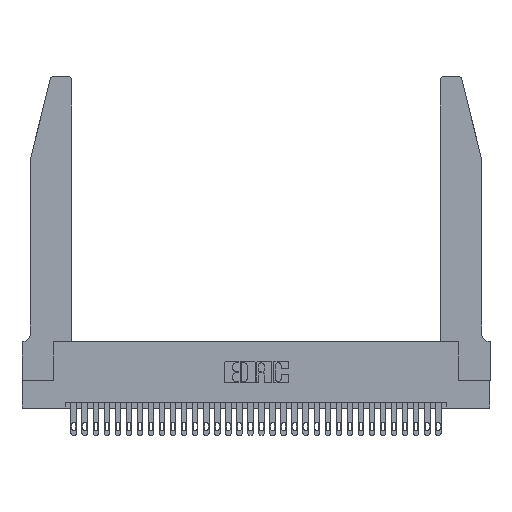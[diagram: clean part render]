
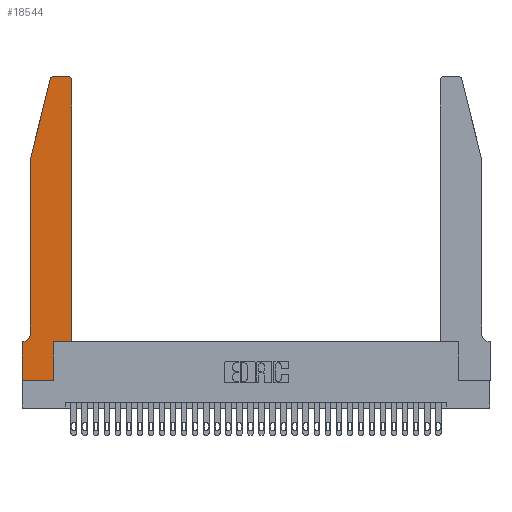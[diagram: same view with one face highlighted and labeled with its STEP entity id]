
A CAD part, top view. The second image highlights one B-rep face of the part: STEP entity #18544.
In plain terms, the highlighted planar face has unit normal (0, 0, 1).
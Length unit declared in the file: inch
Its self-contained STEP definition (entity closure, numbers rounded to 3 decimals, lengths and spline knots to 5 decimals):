
#25 = ORIENTED_EDGE ( 'NONE', *, *, #25476, .T. ) ;
#168 = AXIS2_PLACEMENT_3D ( 'NONE', #1321, #31661, #31769 ) ;
#271 = DIRECTION ( 'NONE',  ( 0., 0., 1. ) ) ;
#1321 = CARTESIAN_POINT ( 'NONE',  ( 0., 0.35, 0.37 ) ) ;
#1745 = VERTEX_POINT ( 'NONE', #8713 ) ;
#1858 = CARTESIAN_POINT ( 'NONE',  ( 0.4505, 2.72, 0.37 ) ) ;
#2359 = EDGE_CURVE ( 'NONE', #8991, #23060, #26266, .T. ) ;
#2499 = LINE ( 'NONE', #14988, #24441 ) ;
#2896 = ORIENTED_EDGE ( 'NONE', *, *, #8494, .T. ) ;
#3615 = DIRECTION ( 'NONE',  ( 1., 0., 0. ) ) ;
#3685 = ORIENTED_EDGE ( 'NONE', *, *, #18693, .T. ) ;
#4271 = CARTESIAN_POINT ( 'NONE',  ( 0.2605, 2.75, 0.37 ) ) ;
#4731 = VECTOR ( 'NONE', #11749, 39.37008 ) ;
#4778 = VERTEX_POINT ( 'NONE', #31301 ) ;
#5156 = CARTESIAN_POINT ( 'NONE',  ( 0.0055, 0.42, 0.37 ) ) ;
#6467 = CARTESIAN_POINT ( 'NONE',  ( 0.0755, 0.35, 0.37 ) ) ;
#7133 = CIRCLE ( 'NONE', #19119, 0.03 ) ;
#7186 = DIRECTION ( 'NONE',  ( 0., -1., 0. ) ) ;
#7257 = CARTESIAN_POINT ( 'NONE',  ( 0.2865, 0.35, 0.37 ) ) ;
#7269 = ORIENTED_EDGE ( 'NONE', *, *, #18301, .T. ) ;
#7534 = CARTESIAN_POINT ( 'NONE',  ( 0.4205, 2.72, 0.37 ) ) ;
#7924 = VERTEX_POINT ( 'NONE', #23741 ) ;
#8092 = CARTESIAN_POINT ( 'NONE',  ( 0.284, 2.72, 0.37 ) ) ;
#8243 = VERTEX_POINT ( 'NONE', #7257 ) ;
#8494 = EDGE_CURVE ( 'NONE', #1745, #23053, #29633, .T. ) ;
#8578 = AXIS2_PLACEMENT_3D ( 'NONE', #7534, #271, #14889 ) ;
#8713 = CARTESIAN_POINT ( 'NONE',  ( 0.0055, 0.35, 0.37 ) ) ;
#8819 = CARTESIAN_POINT ( 'NONE',  ( 0.4505, 0.35, 0.37 ) ) ;
#8991 = VERTEX_POINT ( 'NONE', #28957 ) ;
#9168 = ORIENTED_EDGE ( 'NONE', *, *, #27888, .T. ) ;
#9674 = CIRCLE ( 'NONE', #29770, 0.07 ) ;
#10030 = FACE_OUTER_BOUND ( 'NONE', #10516, .T. ) ;
#10516 = EDGE_LOOP ( 'NONE', ( #11711, #15604, #7269, #23834, #25, #2896, #9168, #18873, #19729, #15677, #13656, #3685 ) ) ;
#10691 = DIRECTION ( 'NONE',  ( 0., 1., 0. ) ) ;
#10832 = LINE ( 'NONE', #20751, #30089 ) ;
#11139 = EDGE_CURVE ( 'NONE', #21052, #8243, #16527, .T. ) ;
#11711 = ORIENTED_EDGE ( 'NONE', *, *, #19107, .T. ) ;
#11749 = DIRECTION ( 'NONE',  ( 0., 1., 0. ) ) ;
#12768 = CIRCLE ( 'NONE', #8578, 0.03 ) ;
#12860 = EDGE_CURVE ( 'NONE', #4778, #23293, #17988, .T. ) ;
#12916 = DIRECTION ( 'NONE',  ( 1., 0., 0. ) ) ;
#13656 = ORIENTED_EDGE ( 'NONE', *, *, #12860, .T. ) ;
#13884 = VERTEX_POINT ( 'NONE', #25799 ) ;
#14024 = PLANE ( 'NONE',  #168 ) ;
#14514 = CARTESIAN_POINT ( 'NONE',  ( 0., 0., 0.37 ) ) ;
#14839 = CARTESIAN_POINT ( 'NONE',  ( 0.4505, 0.35, 0.37 ) ) ;
#14878 = DIRECTION ( 'NONE',  ( 0., 0., -1. ) ) ;
#14889 = DIRECTION ( 'NONE',  ( 1., 0., 0. ) ) ;
#14988 = CARTESIAN_POINT ( 'NONE',  ( 0., 0., 0.37 ) ) ;
#15604 = ORIENTED_EDGE ( 'NONE', *, *, #18107, .T. ) ;
#15677 = ORIENTED_EDGE ( 'NONE', *, *, #18953, .T. ) ;
#16240 = DIRECTION ( 'NONE',  ( -0.239, -0.971, 0. ) ) ;
#16527 = LINE ( 'NONE', #18614, #26670 ) ;
#17095 = EDGE_CURVE ( 'NONE', #13884, #21052, #2499, .T. ) ;
#17143 = VECTOR ( 'NONE', #26791, 39.37008 ) ;
#17759 = DIRECTION ( 'NONE',  ( 0., 0., 1. ) ) ;
#17988 = LINE ( 'NONE', #14839, #4731 ) ;
#18107 = EDGE_CURVE ( 'NONE', #7924, #21574, #7133, .T. ) ;
#18166 = CARTESIAN_POINT ( 'NONE',  ( 0., 0.35, 0.37 ) ) ;
#18277 = LINE ( 'NONE', #8819, #24189 ) ;
#18301 = EDGE_CURVE ( 'NONE', #21574, #8991, #10832, .T. ) ;
#18382 = CARTESIAN_POINT ( 'NONE',  ( 0.2865, 0., 0.37 ) ) ;
#18544 = ADVANCED_FACE ( 'NONE', ( #10030 ), #14024, .T. ) ;
#18614 = CARTESIAN_POINT ( 'NONE',  ( 0.2865, 0.35, 0.37 ) ) ;
#18693 = EDGE_CURVE ( 'NONE', #23293, #31866, #12768, .T. ) ;
#18873 = ORIENTED_EDGE ( 'NONE', *, *, #17095, .T. ) ;
#18953 = EDGE_CURVE ( 'NONE', #8243, #4778, #18277, .T. ) ;
#19107 = EDGE_CURVE ( 'NONE', #31866, #7924, #21092, .T. ) ;
#19119 = AXIS2_PLACEMENT_3D ( 'NONE', #8092, #17759, #12916 ) ;
#19460 = VECTOR ( 'NONE', #28913, 39.37008 ) ;
#19729 = ORIENTED_EDGE ( 'NONE', *, *, #11139, .T. ) ;
#20263 = DIRECTION ( 'NONE',  ( -1., 0., 0. ) ) ;
#20751 = CARTESIAN_POINT ( 'NONE',  ( 0.0755, 2., 0.37 ) ) ;
#21052 = VERTEX_POINT ( 'NONE', #18382 ) ;
#21092 = LINE ( 'NONE', #4271, #17143 ) ;
#21574 = VERTEX_POINT ( 'NONE', #32297 ) ;
#21785 = DIRECTION ( 'NONE',  ( 0., -1., 0. ) ) ;
#22667 = DIRECTION ( 'NONE',  ( 1., 0., 0. ) ) ;
#23053 = VERTEX_POINT ( 'NONE', #18166 ) ;
#23060 = VERTEX_POINT ( 'NONE', #23453 ) ;
#23169 = VECTOR ( 'NONE', #21785, 39.37008 ) ;
#23293 = VERTEX_POINT ( 'NONE', #1858 ) ;
#23453 = CARTESIAN_POINT ( 'NONE',  ( 0.0755, 0.42, 0.37 ) ) ;
#23741 = CARTESIAN_POINT ( 'NONE',  ( 0.284, 2.75, 0.37 ) ) ;
#23834 = ORIENTED_EDGE ( 'NONE', *, *, #2359, .T. ) ;
#24189 = VECTOR ( 'NONE', #3615, 39.37008 ) ;
#24441 = VECTOR ( 'NONE', #22667, 39.37008 ) ;
#25476 = EDGE_CURVE ( 'NONE', #23060, #1745, #9674, .T. ) ;
#25799 = CARTESIAN_POINT ( 'NONE',  ( 0., 0., 0.37 ) ) ;
#26266 = LINE ( 'NONE', #28735, #23169 ) ;
#26382 = VECTOR ( 'NONE', #7186, 39.37008 ) ;
#26670 = VECTOR ( 'NONE', #10691, 39.37008 ) ;
#26791 = DIRECTION ( 'NONE',  ( -1., 0., 0. ) ) ;
#27888 = EDGE_CURVE ( 'NONE', #23053, #13884, #29929, .T. ) ;
#28735 = CARTESIAN_POINT ( 'NONE',  ( 0.0755, 2., 0.37 ) ) ;
#28913 = DIRECTION ( 'NONE',  ( -1., 0., 0. ) ) ;
#28957 = CARTESIAN_POINT ( 'NONE',  ( 0.0755, 2., 0.37 ) ) ;
#29633 = LINE ( 'NONE', #6467, #19460 ) ;
#29770 = AXIS2_PLACEMENT_3D ( 'NONE', #5156, #14878, #20263 ) ;
#29929 = LINE ( 'NONE', #14514, #26382 ) ;
#30089 = VECTOR ( 'NONE', #16240, 39.37008 ) ;
#31301 = CARTESIAN_POINT ( 'NONE',  ( 0.4505, 0.35, 0.37 ) ) ;
#31661 = DIRECTION ( 'NONE',  ( 0., 0., 1. ) ) ;
#31769 = DIRECTION ( 'NONE',  ( 1., 0., 0. ) ) ;
#31866 = VERTEX_POINT ( 'NONE', #32421 ) ;
#32297 = CARTESIAN_POINT ( 'NONE',  ( 0.25487, 2.72718, 0.37 ) ) ;
#32421 = CARTESIAN_POINT ( 'NONE',  ( 0.4205, 2.75, 0.37 ) ) ;
